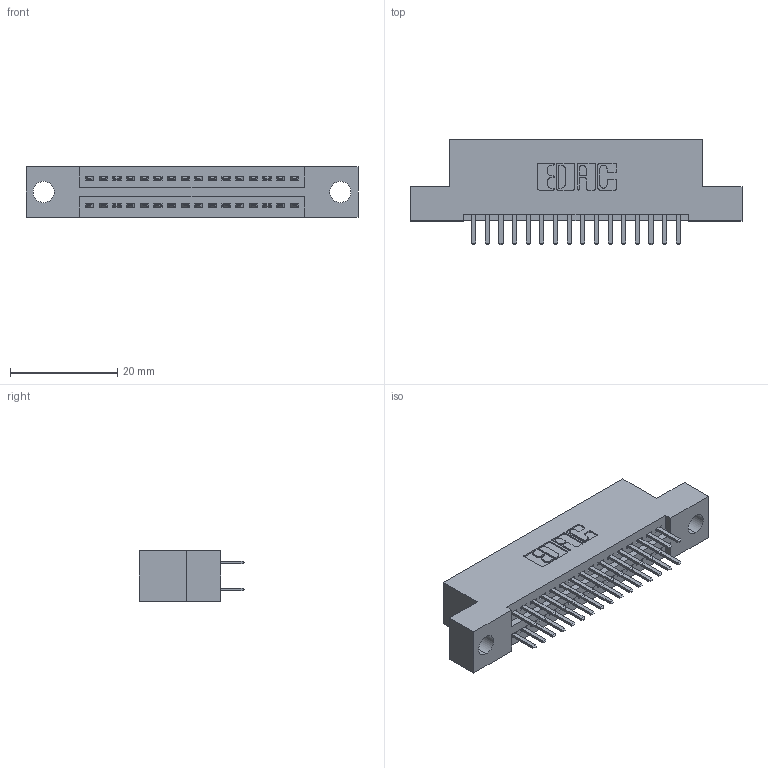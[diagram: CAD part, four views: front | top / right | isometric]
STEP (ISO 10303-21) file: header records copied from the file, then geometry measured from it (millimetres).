
FILE_DESCRIPTION (( 'STEP AP203' ), '1' );
FILE_NAME ('395-032-520-204.STEP', '2021-06-16T20:20:20', ( '' ), ( '' ), 'SwSTEP 2.0', 'SolidWorks 2020', '' );
FILE_SCHEMA (( 'CONFIG_CONTROL_DESIGN' ));
Length unit declared in the file: inch
Products named in the file (3): 345-292-001_345-293-120; 345 Part_Flush Mounting Lugs - 0.156 Dia-TI; 395-032-520-204
Assembly tree (33 placements, depth 2):
  395-032-520-204
    345 Part_Flush Mounting Lugs - 0.156 Dia-TI
    345-292-001_345-293-120  x32
Bounding box: 61.85 x 19.68 x 9.4 mm (x, y, z)
Volume: 5646.7 mm3; surface area: 7664.9 mm2
Topology: 33 solids, 33 shells, 1868 faces, 5401 edges, 3514 vertices
Faces by surface type: plane 1214, cylinder 654
Entity records: 16587 total; most frequent: CARTESIAN_POINT 2822, ORIENTED_EDGE 2742, DIRECTION 2507, EDGE_CURVE 1371, LINE 1171, VECTOR 1171, VERTEX_POINT 910, AXIS2_PLACEMENT_3D 668
